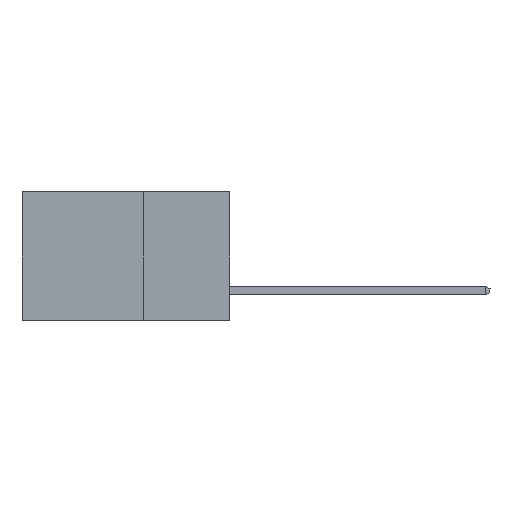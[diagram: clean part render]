
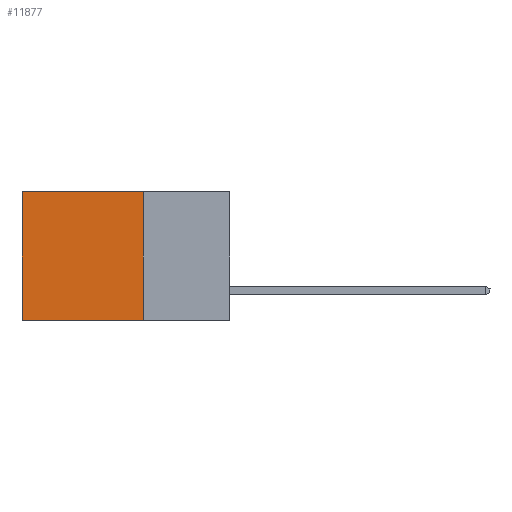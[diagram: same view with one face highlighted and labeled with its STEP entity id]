
A CAD part, left-side view. The second image highlights one B-rep face of the part: STEP entity #11877.
In plain terms, the highlighted planar face has unit normal (-1, 0, 0).
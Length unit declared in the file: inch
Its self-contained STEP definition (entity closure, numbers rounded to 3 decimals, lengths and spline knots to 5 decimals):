
#385 = EDGE_LOOP ( 'NONE', ( #3956, #6192, #5898, #2995 ) ) ;
#811 = VECTOR ( 'NONE', #10612, 39.37008 ) ;
#816 = AXIS2_PLACEMENT_3D ( 'NONE', #15141, #15306, #5010 ) ;
#1218 = DIRECTION ( 'NONE',  ( 0., 0., -1. ) ) ;
#1342 = VERTEX_POINT ( 'NONE', #8300 ) ;
#1690 = CARTESIAN_POINT ( 'NONE',  ( 0.2615, 0.25, -0.37 ) ) ;
#2378 = DIRECTION ( 'NONE',  ( 0., 0., -1. ) ) ;
#2428 = PLANE ( 'NONE',  #816 ) ;
#2995 = ORIENTED_EDGE ( 'NONE', *, *, #3297, .T. ) ;
#3297 = EDGE_CURVE ( 'NONE', #1342, #12637, #5582, .T. ) ;
#3530 = VECTOR ( 'NONE', #2378, 39.37008 ) ;
#3956 = ORIENTED_EDGE ( 'NONE', *, *, #5224, .T. ) ;
#4907 = CARTESIAN_POINT ( 'NONE',  ( 0.2615, 0.25, -0.37 ) ) ;
#4943 = CARTESIAN_POINT ( 'NONE',  ( 0.2615, 0.6, -0.37 ) ) ;
#4973 = VERTEX_POINT ( 'NONE', #9474 ) ;
#5010 = DIRECTION ( 'NONE',  ( 0., 0., -1. ) ) ;
#5133 = DIRECTION ( 'NONE',  ( 0., 1., 0. ) ) ;
#5224 = EDGE_CURVE ( 'NONE', #12637, #5807, #16285, .T. ) ;
#5582 = LINE ( 'NONE', #8253, #811 ) ;
#5807 = VERTEX_POINT ( 'NONE', #4943 ) ;
#5898 = ORIENTED_EDGE ( 'NONE', *, *, #6077, .F. ) ;
#6077 = EDGE_CURVE ( 'NONE', #1342, #4973, #6169, .T. ) ;
#6169 = LINE ( 'NONE', #4907, #9414 ) ;
#6192 = ORIENTED_EDGE ( 'NONE', *, *, #14970, .F. ) ;
#7996 = VECTOR ( 'NONE', #5133, 39.37008 ) ;
#8253 = CARTESIAN_POINT ( 'NONE',  ( 0.2615, 0.25, 0. ) ) ;
#8300 = CARTESIAN_POINT ( 'NONE',  ( 0.2615, 0.25, 0. ) ) ;
#8821 = CARTESIAN_POINT ( 'NONE',  ( 0.2615, 0.6, -0.37 ) ) ;
#9414 = VECTOR ( 'NONE', #1218, 39.37008 ) ;
#9474 = CARTESIAN_POINT ( 'NONE',  ( 0.2615, 0.25, -0.37 ) ) ;
#10214 = FACE_OUTER_BOUND ( 'NONE', #385, .T. ) ;
#10612 = DIRECTION ( 'NONE',  ( 0., 1., 0. ) ) ;
#11877 = ADVANCED_FACE ( 'NONE', ( #10214 ), #2428, .F. ) ;
#12637 = VERTEX_POINT ( 'NONE', #14693 ) ;
#13169 = LINE ( 'NONE', #1690, #7996 ) ;
#14693 = CARTESIAN_POINT ( 'NONE',  ( 0.2615, 0.6, 0. ) ) ;
#14970 = EDGE_CURVE ( 'NONE', #4973, #5807, #13169, .T. ) ;
#15141 = CARTESIAN_POINT ( 'NONE',  ( 0.2615, 0.25, -0.37 ) ) ;
#15306 = DIRECTION ( 'NONE',  ( 1., 0., 0. ) ) ;
#16285 = LINE ( 'NONE', #8821, #3530 ) ;
